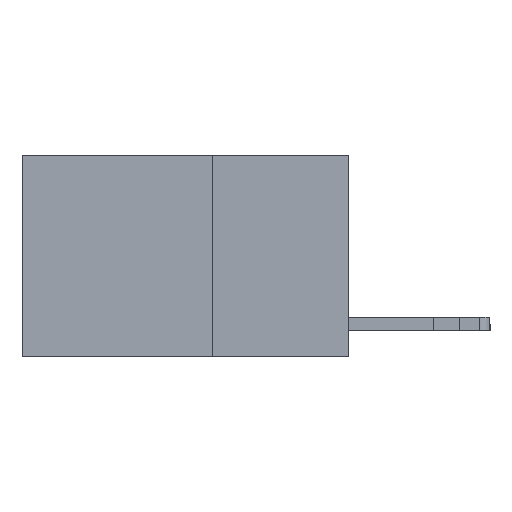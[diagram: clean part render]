
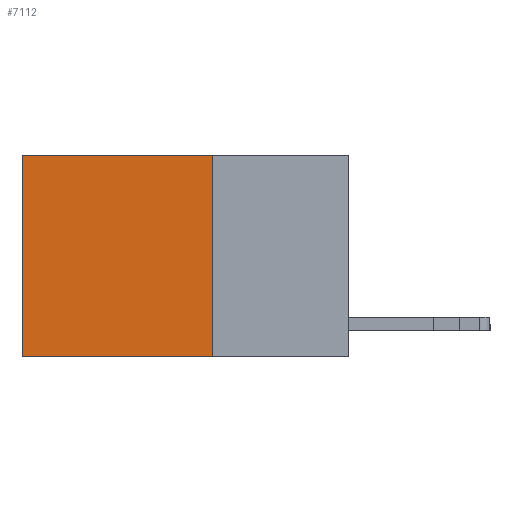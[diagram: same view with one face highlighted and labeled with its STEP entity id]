
A CAD part, left-side view. The second image highlights one B-rep face of the part: STEP entity #7112.
In plain terms, the highlighted planar face has unit normal (-1, 0, 0).
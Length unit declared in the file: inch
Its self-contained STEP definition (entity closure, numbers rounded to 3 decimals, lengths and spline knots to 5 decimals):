
#320 = ORIENTED_EDGE ( 'NONE', *, *, #3393, .F. ) ;
#470 = LINE ( 'NONE', #11317, #21572 ) ;
#570 = EDGE_CURVE ( 'NONE', #2696, #4233, #470, .T. ) ;
#1050 = DIRECTION ( 'NONE',  ( 0., 1., 0. ) ) ;
#1385 = ORIENTED_EDGE ( 'NONE', *, *, #12401, .T. ) ;
#2696 = VERTEX_POINT ( 'NONE', #18691 ) ;
#2956 = LINE ( 'NONE', #21721, #7014 ) ;
#3354 = CARTESIAN_POINT ( 'NONE',  ( 0.2625, 0.25, -0.37 ) ) ;
#3393 = EDGE_CURVE ( 'NONE', #19688, #22004, #2956, .T. ) ;
#4233 = VERTEX_POINT ( 'NONE', #8513 ) ;
#4912 = DIRECTION ( 'NONE',  ( 0., 0., -1. ) ) ;
#7014 = VECTOR ( 'NONE', #4912, 39.37008 ) ;
#7108 = LINE ( 'NONE', #18182, #19126 ) ;
#7112 = ADVANCED_FACE ( 'NONE', ( #7899 ), #22159, .F. ) ;
#7674 = EDGE_LOOP ( 'NONE', ( #18179, #12420, #320, #1385 ) ) ;
#7899 = FACE_OUTER_BOUND ( 'NONE', #7674, .T. ) ;
#8513 = CARTESIAN_POINT ( 'NONE',  ( 0.2625, 0.6, -0.37 ) ) ;
#9069 = DIRECTION ( 'NONE',  ( 0., 1., 0. ) ) ;
#11317 = CARTESIAN_POINT ( 'NONE',  ( 0.2625, 0.6, 0. ) ) ;
#12015 = DIRECTION ( 'NONE',  ( 1., 0., 0. ) ) ;
#12362 = LINE ( 'NONE', #3354, #23324 ) ;
#12401 = EDGE_CURVE ( 'NONE', #19688, #2696, #7108, .T. ) ;
#12420 = ORIENTED_EDGE ( 'NONE', *, *, #22582, .F. ) ;
#13503 = DIRECTION ( 'NONE',  ( 0., 0., -1. ) ) ;
#17065 = CARTESIAN_POINT ( 'NONE',  ( 0.2625, 0.25, 0. ) ) ;
#17477 = CARTESIAN_POINT ( 'NONE',  ( 0.2625, 0.25, 0. ) ) ;
#18179 = ORIENTED_EDGE ( 'NONE', *, *, #570, .T. ) ;
#18182 = CARTESIAN_POINT ( 'NONE',  ( 0.2625, 0.25, 0. ) ) ;
#18691 = CARTESIAN_POINT ( 'NONE',  ( 0.2625, 0.6, 0. ) ) ;
#19126 = VECTOR ( 'NONE', #9069, 39.37008 ) ;
#19460 = DIRECTION ( 'NONE',  ( 0., 0., -1. ) ) ;
#19688 = VERTEX_POINT ( 'NONE', #17065 ) ;
#19801 = AXIS2_PLACEMENT_3D ( 'NONE', #17477, #12015, #19460 ) ;
#21572 = VECTOR ( 'NONE', #13503, 39.37008 ) ;
#21721 = CARTESIAN_POINT ( 'NONE',  ( 0.2625, 0.25, 0. ) ) ;
#22004 = VERTEX_POINT ( 'NONE', #22439 ) ;
#22159 = PLANE ( 'NONE',  #19801 ) ;
#22439 = CARTESIAN_POINT ( 'NONE',  ( 0.2625, 0.25, -0.37 ) ) ;
#22582 = EDGE_CURVE ( 'NONE', #22004, #4233, #12362, .T. ) ;
#23324 = VECTOR ( 'NONE', #1050, 39.37008 ) ;
